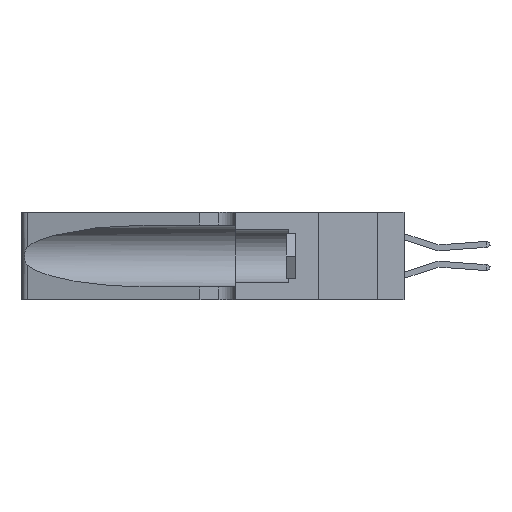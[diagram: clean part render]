
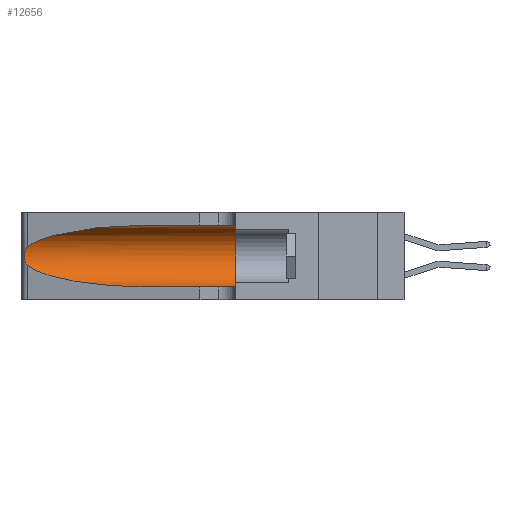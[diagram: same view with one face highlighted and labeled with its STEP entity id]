
A CAD part, left-side view. The second image highlights one B-rep face of the part: STEP entity #12656.
In plain terms, the highlighted cylindrical face has radius 3.308 mm (diameter 6.617 mm), a partial arc.
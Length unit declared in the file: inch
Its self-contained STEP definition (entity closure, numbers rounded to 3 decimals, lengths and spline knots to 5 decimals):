
#1676 = CIRCLE ( 'NONE', #34122, 0.13025 ) ;
#2084 = CARTESIAN_POINT ( 'NONE',  ( 0.1305, 0.72297, 0.31525 ) ) ;
#2185 = CARTESIAN_POINT ( 'NONE',  ( 0.25639, 1.23186, 0.15144 ) ) ;
#2481 =( BOUNDED_CURVE ( )  B_SPLINE_CURVE ( 3, ( #35372, #29700, #24083, #6896 ),
 .UNSPECIFIED., .F., .F. ) 
 B_SPLINE_CURVE_WITH_KNOTS ( ( 4, 4 ),
 ( 3.44316, 4.71239 ),
 .UNSPECIFIED. ) 
 CURVE ( )  GEOMETRIC_REPRESENTATION_ITEM ( )  RATIONAL_B_SPLINE_CURVE ( ( 1., 0.87, 0.87, 1. ) ) 
 REPRESENTATION_ITEM ( '' )  );
#2530 = DIRECTION ( 'NONE',  ( 0., -1., 0. ) ) ;
#4494 = CARTESIAN_POINT ( 'NONE',  ( 0.25487, 1.22718, 0.14631 ) ) ;
#5085 = CARTESIAN_POINT ( 'NONE',  ( 0.25639, 1.23184, 0.21858 ) ) ;
#5145 = CARTESIAN_POINT ( 'NONE',  ( 0.1305, 0.35, 0.185 ) ) ;
#5204 = CARTESIAN_POINT ( 'NONE',  ( 0.25487, 1.22718, 0.14631 ) ) ;
#6503 =( BOUNDED_CURVE ( )  B_SPLINE_CURVE ( 3, ( #10051, #24323, #12922, #32884 ),
 .UNSPECIFIED., .F., .T. ) 
 B_SPLINE_CURVE_WITH_KNOTS ( ( 4, 4 ),
 ( 1.5708, 2.84003 ),
 .UNSPECIFIED. ) 
 CURVE ( )  GEOMETRIC_REPRESENTATION_ITEM ( )  RATIONAL_B_SPLINE_CURVE ( ( 1., 0.87, 0.87, 1. ) ) 
 REPRESENTATION_ITEM ( '' )  );
#6873 = EDGE_CURVE ( 'NONE', #22844, #23851, #35824, .T. ) ;
#6896 = CARTESIAN_POINT ( 'NONE',  ( 0.1305, 0.72297, 0.05475 ) ) ;
#8039 = DIRECTION ( 'NONE',  ( 0., 0., 1. ) ) ;
#8943 = CARTESIAN_POINT ( 'NONE',  ( 0.1305, 1.61858, 0.185 ) ) ;
#9773 = EDGE_CURVE ( 'NONE', #32942, #36098, #20565, .T. ) ;
#10051 = CARTESIAN_POINT ( 'NONE',  ( 0.1305, 0.72297, 0.31525 ) ) ;
#10890 = CARTESIAN_POINT ( 'NONE',  ( 0.25854, 1.2359, 0.20912 ) ) ;
#11115 = CYLINDRICAL_SURFACE ( 'NONE', #27607, 0.13025 ) ;
#12008 = VECTOR ( 'NONE', #17021, 39.37008 ) ;
#12656 = ADVANCED_FACE ( 'NONE', ( #33882 ), #11115, .F. ) ;
#12922 = CARTESIAN_POINT ( 'NONE',  ( 0.2373, 1.15595, 0.28018 ) ) ;
#13781 = CARTESIAN_POINT ( 'NONE',  ( 0.26075, 1.23896, 0.19203 ) ) ;
#14678 = VERTEX_POINT ( 'NONE', #25782 ) ;
#16674 = CARTESIAN_POINT ( 'NONE',  ( 0.26017, 1.23833, 0.17102 ) ) ;
#16826 = ORIENTED_EDGE ( 'NONE', *, *, #9773, .F. ) ;
#16832 = VECTOR ( 'NONE', #2530, 39.37008 ) ;
#16904 = CARTESIAN_POINT ( 'NONE',  ( 0.1305, 1.61858, 0.31525 ) ) ;
#17021 = DIRECTION ( 'NONE',  ( 0., -1., 0. ) ) ;
#17707 = LINE ( 'NONE', #36882, #16832 ) ;
#18361 = CARTESIAN_POINT ( 'NONE',  ( 0.1305, 0.72297, 0.05475 ) ) ;
#19416 = CARTESIAN_POINT ( 'NONE',  ( 0.25555, 1.22994, 0.2215 ) ) ;
#19530 = CARTESIAN_POINT ( 'NONE',  ( 0.25789, 1.23486, 0.15765 ) ) ;
#20565 = LINE ( 'NONE', #16904, #12008 ) ;
#20969 = ORIENTED_EDGE ( 'NONE', *, *, #32398, .F. ) ;
#22445 = CARTESIAN_POINT ( 'NONE',  ( 0.25555, 1.22993, 0.14849 ) ) ;
#22844 = VERTEX_POINT ( 'NONE', #28409 ) ;
#23441 = CARTESIAN_POINT ( 'NONE',  ( 0.1305, 0.35, 0.31525 ) ) ;
#23697 = EDGE_CURVE ( 'NONE', #23851, #36942, #2481, .T. ) ;
#23851 = VERTEX_POINT ( 'NONE', #4494 ) ;
#24083 = CARTESIAN_POINT ( 'NONE',  ( 0.18966, 0.96281, 0.05475 ) ) ;
#24323 = CARTESIAN_POINT ( 'NONE',  ( 0.18966, 0.96281, 0.31525 ) ) ;
#25166 = CARTESIAN_POINT ( 'NONE',  ( 0.25487, 1.22718, 0.22369 ) ) ;
#25235 = DIRECTION ( 'NONE',  ( 0., 1., 0. ) ) ;
#25782 = CARTESIAN_POINT ( 'NONE',  ( 0.1305, 0.35, 0.05475 ) ) ;
#26127 = DIRECTION ( 'NONE',  ( 0., 0., -1. ) ) ;
#27607 = AXIS2_PLACEMENT_3D ( 'NONE', #8943, #28987, #26127 ) ;
#28040 = CARTESIAN_POINT ( 'NONE',  ( 0.25787, 1.23484, 0.2124 ) ) ;
#28409 = CARTESIAN_POINT ( 'NONE',  ( 0.25487, 1.22718, 0.22369 ) ) ;
#28987 = DIRECTION ( 'NONE',  ( 0., -1., 0. ) ) ;
#28998 = ORIENTED_EDGE ( 'NONE', *, *, #6873, .T. ) ;
#29700 = CARTESIAN_POINT ( 'NONE',  ( 0.2373, 1.15595, 0.08982 ) ) ;
#29991 = ORIENTED_EDGE ( 'NONE', *, *, #23697, .T. ) ;
#30407 = ORIENTED_EDGE ( 'NONE', *, *, #30793, .T. ) ;
#30793 = EDGE_CURVE ( 'NONE', #36942, #14678, #17707, .T. ) ;
#30866 = CARTESIAN_POINT ( 'NONE',  ( 0.26018, 1.23835, 0.19895 ) ) ;
#32398 = EDGE_CURVE ( 'NONE', #36098, #14678, #1676, .T. ) ;
#32611 = ORIENTED_EDGE ( 'NONE', *, *, #35698, .T. ) ;
#32884 = CARTESIAN_POINT ( 'NONE',  ( 0.25487, 1.22718, 0.22369 ) ) ;
#32942 = VERTEX_POINT ( 'NONE', #2084 ) ;
#33709 = CARTESIAN_POINT ( 'NONE',  ( 0.26075, 1.23896, 0.178 ) ) ;
#33882 = FACE_OUTER_BOUND ( 'NONE', #34682, .T. ) ;
#34122 = AXIS2_PLACEMENT_3D ( 'NONE', #5145, #25235, #8039 ) ;
#34682 = EDGE_LOOP ( 'NONE', ( #32611, #28998, #29991, #30407, #20969, #16826 ) ) ;
#35372 = CARTESIAN_POINT ( 'NONE',  ( 0.25487, 1.22718, 0.14631 ) ) ;
#35698 = EDGE_CURVE ( 'NONE', #32942, #22844, #6503, .T. ) ;
#35824 = B_SPLINE_CURVE_WITH_KNOTS ( 'NONE', 3,
 ( #25166, #19416, #5085, #28040, #10890, #30866, #13781, #33709, #16674, #36555, #19530, #2185, #22445, #5204 ),
 .UNSPECIFIED., .F., .F.,
 ( 4, 2, 2, 2, 2, 2, 4 ),
 ( 0., 0.00027, 0.00053, 0.00107, 0.0016, 0.00187, 0.00214 ),
 .UNSPECIFIED. ) ;
#36098 = VERTEX_POINT ( 'NONE', #23441 ) ;
#36555 = CARTESIAN_POINT ( 'NONE',  ( 0.25856, 1.23593, 0.16098 ) ) ;
#36882 = CARTESIAN_POINT ( 'NONE',  ( 0.1305, 1.61858, 0.05475 ) ) ;
#36942 = VERTEX_POINT ( 'NONE', #18361 ) ;
